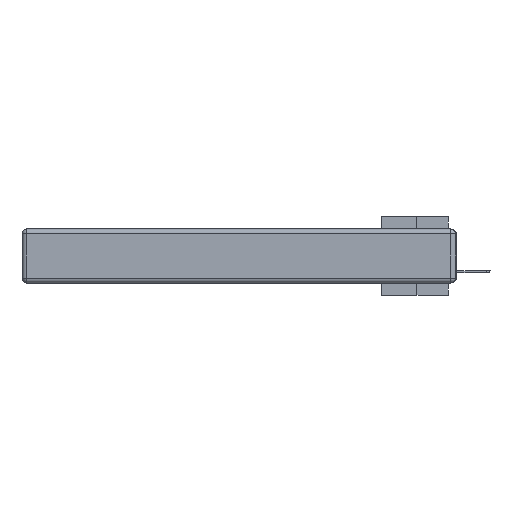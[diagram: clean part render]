
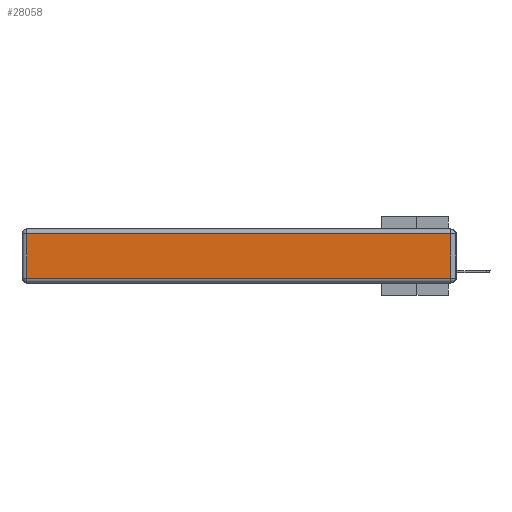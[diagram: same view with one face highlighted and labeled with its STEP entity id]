
A CAD part, left-side view. The second image highlights one B-rep face of the part: STEP entity #28058.
In plain terms, the highlighted planar face has unit normal (-1, 0, 0).
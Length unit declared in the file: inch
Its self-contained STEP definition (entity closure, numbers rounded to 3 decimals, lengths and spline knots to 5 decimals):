
#207 = EDGE_LOOP ( 'NONE', ( #27845, #16189, #18574, #6915 ) ) ;
#238 = PLANE ( 'NONE',  #15722 ) ;
#2500 = VERTEX_POINT ( 'NONE', #18648 ) ;
#4283 = CARTESIAN_POINT ( 'NONE',  ( 0., 2.72, -0.03 ) ) ;
#4723 = CARTESIAN_POINT ( 'NONE',  ( 0., 0.03, -0.03 ) ) ;
#5548 = EDGE_CURVE ( 'NONE', #2500, #14005, #8740, .T. ) ;
#5896 = DIRECTION ( 'NONE',  ( 0., 1., 0. ) ) ;
#6915 = ORIENTED_EDGE ( 'NONE', *, *, #25213, .T. ) ;
#8676 = VERTEX_POINT ( 'NONE', #22776 ) ;
#8740 = LINE ( 'NONE', #13624, #23645 ) ;
#8932 = LINE ( 'NONE', #10571, #24067 ) ;
#10366 = LINE ( 'NONE', #28652, #17539 ) ;
#10571 = CARTESIAN_POINT ( 'NONE',  ( 0., 2.72, -0.343 ) ) ;
#11489 = FACE_OUTER_BOUND ( 'NONE', #207, .T. ) ;
#13250 = DIRECTION ( 'NONE',  ( 0., 0., 1. ) ) ;
#13624 = CARTESIAN_POINT ( 'NONE',  ( 0., 0.03, -0.343 ) ) ;
#14005 = VERTEX_POINT ( 'NONE', #4723 ) ;
#14695 = VECTOR ( 'NONE', #5896, 39.37008 ) ;
#15722 = AXIS2_PLACEMENT_3D ( 'NONE', #18145, #27120, #13250 ) ;
#15845 = DIRECTION ( 'NONE',  ( 0., 0., 1. ) ) ;
#16189 = ORIENTED_EDGE ( 'NONE', *, *, #5548, .T. ) ;
#16706 = EDGE_CURVE ( 'NONE', #8676, #2500, #10366, .T. ) ;
#17539 = VECTOR ( 'NONE', #23644, 39.37008 ) ;
#18145 = CARTESIAN_POINT ( 'NONE',  ( 0., 0., -0.343 ) ) ;
#18574 = ORIENTED_EDGE ( 'NONE', *, *, #24658, .T. ) ;
#18648 = CARTESIAN_POINT ( 'NONE',  ( 0., 0.03, -0.313 ) ) ;
#19345 = LINE ( 'NONE', #28321, #14695 ) ;
#19883 = DIRECTION ( 'NONE',  ( 0., 0., -1. ) ) ;
#22776 = CARTESIAN_POINT ( 'NONE',  ( 0., 2.72, -0.313 ) ) ;
#23644 = DIRECTION ( 'NONE',  ( 0., -1., 0. ) ) ;
#23645 = VECTOR ( 'NONE', #15845, 39.37008 ) ;
#24067 = VECTOR ( 'NONE', #19883, 39.37008 ) ;
#24658 = EDGE_CURVE ( 'NONE', #14005, #27623, #19345, .T. ) ;
#25213 = EDGE_CURVE ( 'NONE', #27623, #8676, #8932, .T. ) ;
#27120 = DIRECTION ( 'NONE',  ( -1., 0., 0. ) ) ;
#27623 = VERTEX_POINT ( 'NONE', #4283 ) ;
#27845 = ORIENTED_EDGE ( 'NONE', *, *, #16706, .T. ) ;
#28058 = ADVANCED_FACE ( 'NONE', ( #11489 ), #238, .T. ) ;
#28321 = CARTESIAN_POINT ( 'NONE',  ( 0., 2.75, -0.03 ) ) ;
#28652 = CARTESIAN_POINT ( 'NONE',  ( 0., 0., -0.313 ) ) ;
